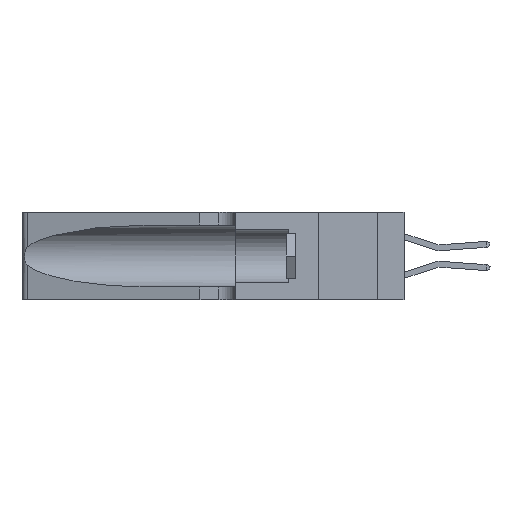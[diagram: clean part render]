
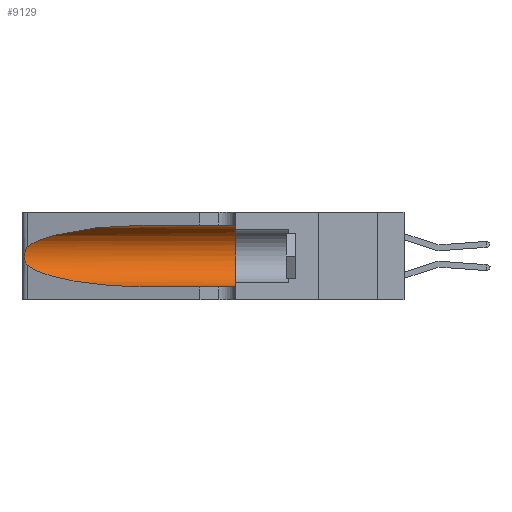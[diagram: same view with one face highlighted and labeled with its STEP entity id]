
A CAD part, left-side view. The second image highlights one B-rep face of the part: STEP entity #9129.
In plain terms, the highlighted cylindrical face has radius 3.308 mm (diameter 6.617 mm), a partial arc.
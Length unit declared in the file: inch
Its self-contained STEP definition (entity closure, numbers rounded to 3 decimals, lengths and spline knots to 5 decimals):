
#281 = CARTESIAN_POINT ( 'NONE',  ( 0.26017, 1.23833, 0.17102 ) ) ;
#492 = FACE_OUTER_BOUND ( 'NONE', #17457, .T. ) ;
#2093 = VERTEX_POINT ( 'NONE', #12053 ) ;
#2569 = CARTESIAN_POINT ( 'NONE',  ( 0.25789, 1.23486, 0.15765 ) ) ;
#2743 = VERTEX_POINT ( 'NONE', #24822 ) ;
#3078 = CARTESIAN_POINT ( 'NONE',  ( 0.2373, 1.15595, 0.28018 ) ) ;
#3575 = VECTOR ( 'NONE', #22751, 39.37008 ) ;
#3679 = EDGE_CURVE ( 'NONE', #2093, #8436, #24345, .T. ) ;
#4872 = CARTESIAN_POINT ( 'NONE',  ( 0.25555, 1.22993, 0.14849 ) ) ;
#5226 = EDGE_CURVE ( 'NONE', #2093, #6174, #16929, .T. ) ;
#5892 = DIRECTION ( 'NONE',  ( 0., -1., 0. ) ) ;
#6174 = VERTEX_POINT ( 'NONE', #26416 ) ;
#6300 = ORIENTED_EDGE ( 'NONE', *, *, #11503, .T. ) ;
#6753 = CARTESIAN_POINT ( 'NONE',  ( 0.1305, 0.72297, 0.05475 ) ) ;
#7349 = CARTESIAN_POINT ( 'NONE',  ( 0.25487, 1.22718, 0.14631 ) ) ;
#7770 = ORIENTED_EDGE ( 'NONE', *, *, #24113, .T. ) ;
#7932 = CARTESIAN_POINT ( 'NONE',  ( 0.25487, 1.22718, 0.14631 ) ) ;
#8436 = VERTEX_POINT ( 'NONE', #15906 ) ;
#9051 = EDGE_CURVE ( 'NONE', #8436, #12273, #14405, .T. ) ;
#9129 = ADVANCED_FACE ( 'NONE', ( #492 ), #11723, .F. ) ;
#9255 = CARTESIAN_POINT ( 'NONE',  ( 0.25787, 1.23484, 0.2124 ) ) ;
#9571 = CARTESIAN_POINT ( 'NONE',  ( 0.18966, 0.96281, 0.05475 ) ) ;
#9747 = CARTESIAN_POINT ( 'NONE',  ( 0.1305, 0.72297, 0.31525 ) ) ;
#11222 = VECTOR ( 'NONE', #5892, 39.37008 ) ;
#11421 = CARTESIAN_POINT ( 'NONE',  ( 0.1305, 0.35, 0.185 ) ) ;
#11470 = CARTESIAN_POINT ( 'NONE',  ( 0.26018, 1.23835, 0.19895 ) ) ;
#11503 = EDGE_CURVE ( 'NONE', #13104, #2743, #20974, .T. ) ;
#11723 = CYLINDRICAL_SURFACE ( 'NONE', #16807, 0.13025 ) ;
#11741 = DIRECTION ( 'NONE',  ( 0., 0., -1. ) ) ;
#12053 = CARTESIAN_POINT ( 'NONE',  ( 0.1305, 0.72297, 0.31525 ) ) ;
#12273 = VERTEX_POINT ( 'NONE', #7932 ) ;
#12681 = ORIENTED_EDGE ( 'NONE', *, *, #17822, .F. ) ;
#13104 = VERTEX_POINT ( 'NONE', #6753 ) ;
#13520 = CARTESIAN_POINT ( 'NONE',  ( 0.25555, 1.22994, 0.2215 ) ) ;
#13553 = DIRECTION ( 'NONE',  ( 0., 0., 1. ) ) ;
#13602 = CARTESIAN_POINT ( 'NONE',  ( 0.26075, 1.23896, 0.178 ) ) ;
#13870 = DIRECTION ( 'NONE',  ( 0., -1., 0. ) ) ;
#13876 = ORIENTED_EDGE ( 'NONE', *, *, #3679, .T. ) ;
#13982 = CARTESIAN_POINT ( 'NONE',  ( 0.18966, 0.96281, 0.31525 ) ) ;
#14405 = B_SPLINE_CURVE_WITH_KNOTS ( 'NONE', 3,
 ( #15683, #13520, #22117, #9255, #24264, #11470, #26425, #13602, #281, #15777, #2569, #17932, #4872, #20078 ),
 .UNSPECIFIED., .F., .F.,
 ( 4, 2, 2, 2, 2, 2, 4 ),
 ( 0., 0.00027, 0.00053, 0.00107, 0.0016, 0.00187, 0.00214 ),
 .UNSPECIFIED. ) ;
#14697 = ORIENTED_EDGE ( 'NONE', *, *, #5226, .F. ) ;
#15683 = CARTESIAN_POINT ( 'NONE',  ( 0.25487, 1.22718, 0.22369 ) ) ;
#15777 = CARTESIAN_POINT ( 'NONE',  ( 0.25856, 1.23593, 0.16098 ) ) ;
#15906 = CARTESIAN_POINT ( 'NONE',  ( 0.25487, 1.22718, 0.22369 ) ) ;
#16807 = AXIS2_PLACEMENT_3D ( 'NONE', #26697, #13870, #11741 ) ;
#16929 = LINE ( 'NONE', #21051, #11222 ) ;
#17338 =( BOUNDED_CURVE ( )  B_SPLINE_CURVE ( 3, ( #7349, #22430, #9571, #24577 ),
 .UNSPECIFIED., .F., .T. ) 
 B_SPLINE_CURVE_WITH_KNOTS ( ( 4, 4 ),
 ( 3.44316, 4.71239 ),
 .UNSPECIFIED. ) 
 CURVE ( )  GEOMETRIC_REPRESENTATION_ITEM ( )  RATIONAL_B_SPLINE_CURVE ( ( 1., 0.87, 0.87, 1. ) ) 
 REPRESENTATION_ITEM ( '' )  );
#17457 = EDGE_LOOP ( 'NONE', ( #13876, #20576, #7770, #6300, #12681, #14697 ) ) ;
#17822 = EDGE_CURVE ( 'NONE', #6174, #2743, #24456, .T. ) ;
#17932 = CARTESIAN_POINT ( 'NONE',  ( 0.25639, 1.23186, 0.15144 ) ) ;
#18422 = CARTESIAN_POINT ( 'NONE',  ( 0.25487, 1.22718, 0.22369 ) ) ;
#20078 = CARTESIAN_POINT ( 'NONE',  ( 0.25487, 1.22718, 0.14631 ) ) ;
#20576 = ORIENTED_EDGE ( 'NONE', *, *, #9051, .T. ) ;
#20625 = CARTESIAN_POINT ( 'NONE',  ( 0.1305, 1.61858, 0.05475 ) ) ;
#20974 = LINE ( 'NONE', #20625, #3575 ) ;
#21051 = CARTESIAN_POINT ( 'NONE',  ( 0.1305, 1.61858, 0.31525 ) ) ;
#22117 = CARTESIAN_POINT ( 'NONE',  ( 0.25639, 1.23184, 0.21858 ) ) ;
#22430 = CARTESIAN_POINT ( 'NONE',  ( 0.2373, 1.15595, 0.08982 ) ) ;
#22751 = DIRECTION ( 'NONE',  ( 0., -1., 0. ) ) ;
#24113 = EDGE_CURVE ( 'NONE', #12273, #13104, #17338, .T. ) ;
#24264 = CARTESIAN_POINT ( 'NONE',  ( 0.25854, 1.2359, 0.20912 ) ) ;
#24345 =( BOUNDED_CURVE ( )  B_SPLINE_CURVE ( 3, ( #9747, #13982, #3078, #18422 ),
 .UNSPECIFIED., .F., .F. ) 
 B_SPLINE_CURVE_WITH_KNOTS ( ( 4, 4 ),
 ( 1.5708, 2.84003 ),
 .UNSPECIFIED. ) 
 CURVE ( )  GEOMETRIC_REPRESENTATION_ITEM ( )  RATIONAL_B_SPLINE_CURVE ( ( 1., 0.87, 0.87, 1. ) ) 
 REPRESENTATION_ITEM ( '' )  );
#24456 = CIRCLE ( 'NONE', #27119, 0.13025 ) ;
#24577 = CARTESIAN_POINT ( 'NONE',  ( 0.1305, 0.72297, 0.05475 ) ) ;
#24822 = CARTESIAN_POINT ( 'NONE',  ( 0.1305, 0.35, 0.05475 ) ) ;
#26377 = DIRECTION ( 'NONE',  ( 0., 1., 0. ) ) ;
#26416 = CARTESIAN_POINT ( 'NONE',  ( 0.1305, 0.35, 0.31525 ) ) ;
#26425 = CARTESIAN_POINT ( 'NONE',  ( 0.26075, 1.23896, 0.19203 ) ) ;
#26697 = CARTESIAN_POINT ( 'NONE',  ( 0.1305, 1.61858, 0.185 ) ) ;
#27119 = AXIS2_PLACEMENT_3D ( 'NONE', #11421, #26377, #13553 ) ;
